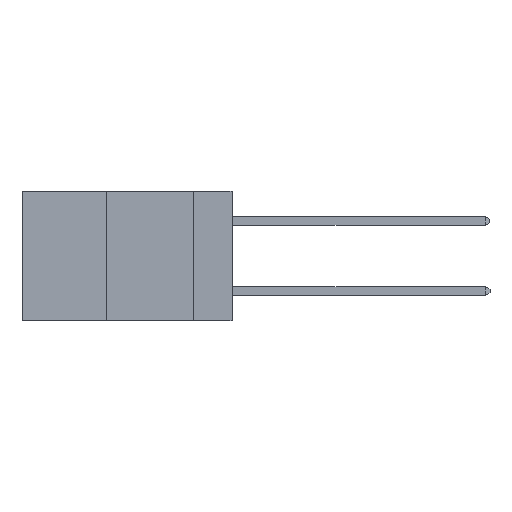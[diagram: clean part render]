
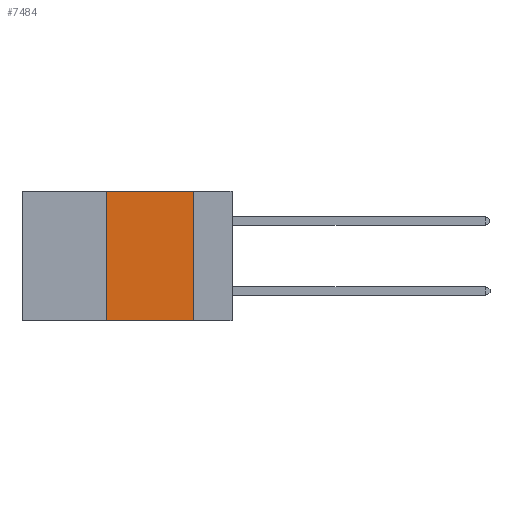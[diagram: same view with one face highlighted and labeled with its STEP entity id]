
A CAD part, left-side view. The second image highlights one B-rep face of the part: STEP entity #7484.
In plain terms, the highlighted planar face has unit normal (-1, 0, 0).
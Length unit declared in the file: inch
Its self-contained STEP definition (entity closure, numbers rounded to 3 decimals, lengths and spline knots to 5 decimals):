
#155 = ORIENTED_EDGE ( 'NONE', *, *, #17766, .F. ) ;
#469 = ORIENTED_EDGE ( 'NONE', *, *, #8515, .F. ) ;
#835 = ORIENTED_EDGE ( 'NONE', *, *, #18588, .T. ) ;
#840 = VECTOR ( 'NONE', #10347, 39.37008 ) ;
#1086 = DIRECTION ( 'NONE',  ( 0., 0., -1. ) ) ;
#2887 = DIRECTION ( 'NONE',  ( 0., 0., -1. ) ) ;
#3137 = LINE ( 'NONE', #17855, #20771 ) ;
#4350 = DIRECTION ( 'NONE',  ( 0., 0., 1. ) ) ;
#4559 = VERTEX_POINT ( 'NONE', #14461 ) ;
#5512 = VECTOR ( 'NONE', #1086, 39.37008 ) ;
#5940 = VECTOR ( 'NONE', #4350, 39.37008 ) ;
#7166 = DIRECTION ( 'NONE',  ( 0., -1., 0. ) ) ;
#7484 = ADVANCED_FACE ( 'NONE', ( #10975 ), #22201, .F. ) ;
#8224 = VERTEX_POINT ( 'NONE', #14135 ) ;
#8515 = EDGE_CURVE ( 'NONE', #8224, #17223, #10639, .T. ) ;
#10347 = DIRECTION ( 'NONE',  ( 0., -1., 0. ) ) ;
#10639 = LINE ( 'NONE', #13210, #5940 ) ;
#10975 = FACE_OUTER_BOUND ( 'NONE', #14149, .T. ) ;
#11023 = CARTESIAN_POINT ( 'NONE',  ( 0., 0.36, 0. ) ) ;
#11819 = CARTESIAN_POINT ( 'NONE',  ( 0., 0.6, 0. ) ) ;
#11885 = CARTESIAN_POINT ( 'NONE',  ( 0., 0.11, 0. ) ) ;
#12193 = CARTESIAN_POINT ( 'NONE',  ( 0., 0.6, 0. ) ) ;
#12305 = EDGE_CURVE ( 'NONE', #4559, #13413, #18995, .T. ) ;
#13000 = CARTESIAN_POINT ( 'NONE',  ( 0., 0.11, -0.37 ) ) ;
#13210 = CARTESIAN_POINT ( 'NONE',  ( 0., 0.36, 0. ) ) ;
#13413 = VERTEX_POINT ( 'NONE', #13000 ) ;
#13614 = DIRECTION ( 'NONE',  ( 1., 0., 0. ) ) ;
#13707 = ORIENTED_EDGE ( 'NONE', *, *, #12305, .F. ) ;
#14135 = CARTESIAN_POINT ( 'NONE',  ( 0., 0.36, -0.37 ) ) ;
#14149 = EDGE_LOOP ( 'NONE', ( #13707, #155, #469, #835 ) ) ;
#14461 = CARTESIAN_POINT ( 'NONE',  ( 0., 0.11, 0. ) ) ;
#15780 = AXIS2_PLACEMENT_3D ( 'NONE', #11819, #13614, #2887 ) ;
#17223 = VERTEX_POINT ( 'NONE', #11023 ) ;
#17766 = EDGE_CURVE ( 'NONE', #17223, #4559, #19743, .T. ) ;
#17855 = CARTESIAN_POINT ( 'NONE',  ( 0., 0.6, -0.37 ) ) ;
#18588 = EDGE_CURVE ( 'NONE', #8224, #13413, #3137, .T. ) ;
#18995 = LINE ( 'NONE', #11885, #5512 ) ;
#19743 = LINE ( 'NONE', #12193, #840 ) ;
#20771 = VECTOR ( 'NONE', #7166, 39.37008 ) ;
#22201 = PLANE ( 'NONE',  #15780 ) ;
